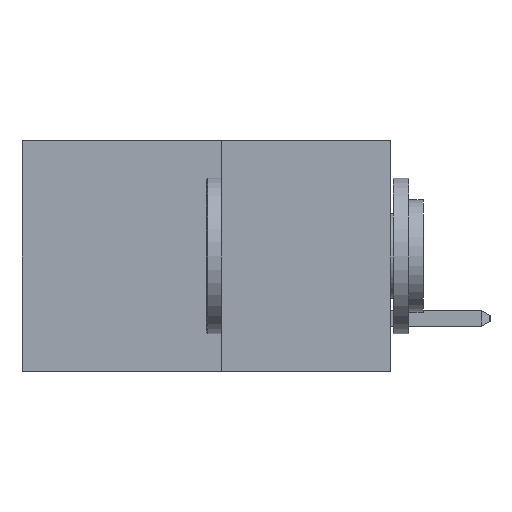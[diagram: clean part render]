
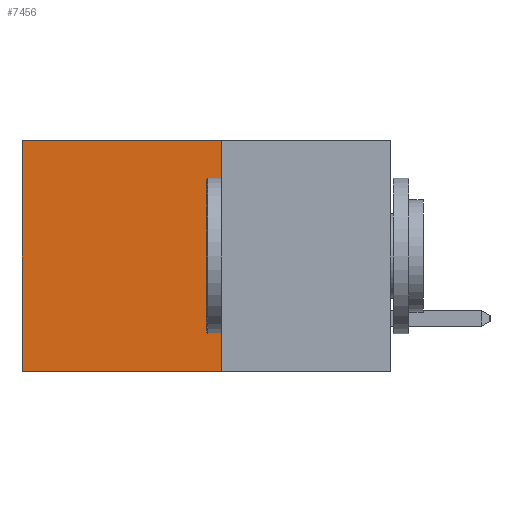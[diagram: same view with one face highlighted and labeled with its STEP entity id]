
A CAD part, left-side view. The second image highlights one B-rep face of the part: STEP entity #7456.
In plain terms, the highlighted planar face has unit normal (-1, 0, 0).
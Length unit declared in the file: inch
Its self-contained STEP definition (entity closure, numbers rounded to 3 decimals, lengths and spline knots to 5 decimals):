
#837 = EDGE_CURVE ( 'NONE', #10995, #11232, #5521, .T. ) ;
#1234 = CARTESIAN_POINT ( 'NONE',  ( 0.277, 0.59, -0.37 ) ) ;
#1421 = VERTEX_POINT ( 'NONE', #7001 ) ;
#1716 = AXIS2_PLACEMENT_3D ( 'NONE', #8231, #10891, #5469 ) ;
#1893 = DIRECTION ( 'NONE',  ( 0., 1., 0. ) ) ;
#2492 = ORIENTED_EDGE ( 'NONE', *, *, #6497, .F. ) ;
#2588 = LINE ( 'NONE', #8411, #9568 ) ;
#2716 = PLANE ( 'NONE',  #1716 ) ;
#3186 = ORIENTED_EDGE ( 'NONE', *, *, #837, .T. ) ;
#3448 = LINE ( 'NONE', #10955, #8082 ) ;
#4668 = CARTESIAN_POINT ( 'NONE',  ( 0.277, 0.27, -0.37 ) ) ;
#4678 = DIRECTION ( 'NONE',  ( 0., 0., -1. ) ) ;
#5469 = DIRECTION ( 'NONE',  ( 0., 0., -1. ) ) ;
#5521 = LINE ( 'NONE', #11264, #9803 ) ;
#5629 = DIRECTION ( 'NONE',  ( 0., 1., 0. ) ) ;
#6455 = CARTESIAN_POINT ( 'NONE',  ( 0.277, 0.59, 0. ) ) ;
#6497 = EDGE_CURVE ( 'NONE', #1421, #7849, #2588, .T. ) ;
#6769 = FACE_OUTER_BOUND ( 'NONE', #8151, .T. ) ;
#7001 = CARTESIAN_POINT ( 'NONE',  ( 0.277, 0.27, 0. ) ) ;
#7456 = ADVANCED_FACE ( 'NONE', ( #6769 ), #2716, .F. ) ;
#7678 = ORIENTED_EDGE ( 'NONE', *, *, #11023, .T. ) ;
#7849 = VERTEX_POINT ( 'NONE', #8724 ) ;
#8082 = VECTOR ( 'NONE', #1893, 39.37008 ) ;
#8151 = EDGE_LOOP ( 'NONE', ( #3186, #8937, #2492, #7678 ) ) ;
#8231 = CARTESIAN_POINT ( 'NONE',  ( 0.277, 0.27, -0.37 ) ) ;
#8237 = LINE ( 'NONE', #4668, #10301 ) ;
#8411 = CARTESIAN_POINT ( 'NONE',  ( 0.277, 0.27, -0.37 ) ) ;
#8724 = CARTESIAN_POINT ( 'NONE',  ( 0.277, 0.27, -0.37 ) ) ;
#8937 = ORIENTED_EDGE ( 'NONE', *, *, #10442, .F. ) ;
#9376 = DIRECTION ( 'NONE',  ( 0., 0., -1. ) ) ;
#9568 = VECTOR ( 'NONE', #9376, 39.37008 ) ;
#9803 = VECTOR ( 'NONE', #4678, 39.37008 ) ;
#10301 = VECTOR ( 'NONE', #5629, 39.37008 ) ;
#10442 = EDGE_CURVE ( 'NONE', #7849, #11232, #8237, .T. ) ;
#10891 = DIRECTION ( 'NONE',  ( 1., 0., 0. ) ) ;
#10955 = CARTESIAN_POINT ( 'NONE',  ( 0.277, 0.27, 0. ) ) ;
#10995 = VERTEX_POINT ( 'NONE', #6455 ) ;
#11023 = EDGE_CURVE ( 'NONE', #1421, #10995, #3448, .T. ) ;
#11232 = VERTEX_POINT ( 'NONE', #1234 ) ;
#11264 = CARTESIAN_POINT ( 'NONE',  ( 0.277, 0.59, -0.37 ) ) ;
